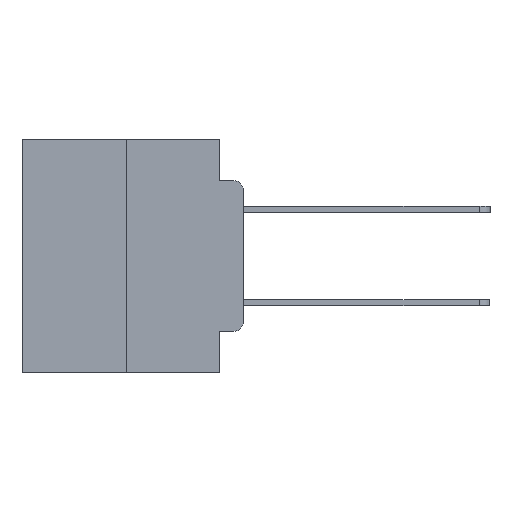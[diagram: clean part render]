
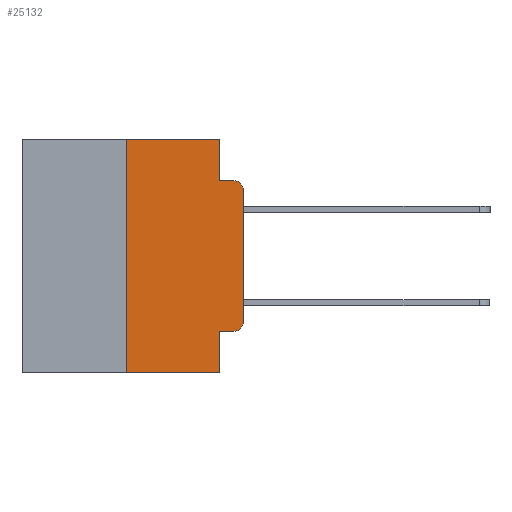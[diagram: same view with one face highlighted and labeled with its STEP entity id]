
A CAD part, left-side view. The second image highlights one B-rep face of the part: STEP entity #25132.
In plain terms, the highlighted planar face has unit normal (-1, 0, 0).
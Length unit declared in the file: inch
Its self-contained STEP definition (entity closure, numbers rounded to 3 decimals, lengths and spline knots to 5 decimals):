
#66 = CARTESIAN_POINT ( 'NONE',  ( 0., 0.051, -0.5 ) ) ;
#108 = CARTESIAN_POINT ( 'NONE',  ( 0., 0.02, -0.1085 ) ) ;
#1156 = ORIENTED_EDGE ( 'NONE', *, *, #16213, .T. ) ;
#1278 = FACE_OUTER_BOUND ( 'NONE', #3934, .T. ) ;
#1354 = VECTOR ( 'NONE', #22344, 39.37008 ) ;
#2232 = VECTOR ( 'NONE', #16869, 39.37008 ) ;
#2329 = DIRECTION ( 'NONE',  ( 0., 0., -1. ) ) ;
#2457 = EDGE_CURVE ( 'NONE', #13263, #21846, #18637, .T. ) ;
#3213 = CARTESIAN_POINT ( 'NONE',  ( 0., 0.02, -0.3915 ) ) ;
#3275 = CARTESIAN_POINT ( 'NONE',  ( 0., 0.051, -0.4115 ) ) ;
#3934 = EDGE_LOOP ( 'NONE', ( #9093, #15205, #4884, #15850, #16503, #17152, #1156, #7487, #18450, #19098 ) ) ;
#4312 = CIRCLE ( 'NONE', #15106, 0.02 ) ;
#4454 = CARTESIAN_POINT ( 'NONE',  ( 0., 0.25, -0.5 ) ) ;
#4498 = DIRECTION ( 'NONE',  ( 0., 0., 1. ) ) ;
#4884 = ORIENTED_EDGE ( 'NONE', *, *, #15669, .F. ) ;
#5142 = CARTESIAN_POINT ( 'NONE',  ( 0., 0., 0. ) ) ;
#5264 = CARTESIAN_POINT ( 'NONE',  ( 0., 0.473, -0.5 ) ) ;
#5349 = DIRECTION ( 'NONE',  ( 0., 0., -1. ) ) ;
#5828 = VERTEX_POINT ( 'NONE', #8620 ) ;
#6153 = DIRECTION ( 'NONE',  ( 0., -1., 0. ) ) ;
#6256 = CIRCLE ( 'NONE', #11082, 0.02 ) ;
#6885 = EDGE_CURVE ( 'NONE', #24458, #19609, #12962, .T. ) ;
#7334 = VECTOR ( 'NONE', #21661, 39.37008 ) ;
#7487 = ORIENTED_EDGE ( 'NONE', *, *, #10504, .F. ) ;
#7636 = CARTESIAN_POINT ( 'NONE',  ( 0., 0.051, -0.0885 ) ) ;
#7838 = LINE ( 'NONE', #25071, #2232 ) ;
#8212 = EDGE_CURVE ( 'NONE', #26313, #9872, #26751, .T. ) ;
#8465 = DIRECTION ( 'NONE',  ( 0., -1., 0. ) ) ;
#8620 = CARTESIAN_POINT ( 'NONE',  ( 0., 0.02, -0.0885 ) ) ;
#8842 = VERTEX_POINT ( 'NONE', #4454 ) ;
#8914 = VECTOR ( 'NONE', #21525, 39.37008 ) ;
#9093 = ORIENTED_EDGE ( 'NONE', *, *, #6885, .T. ) ;
#9577 = LINE ( 'NONE', #21605, #8914 ) ;
#9722 = DIRECTION ( 'NONE',  ( 0., 0., -1. ) ) ;
#9872 = VERTEX_POINT ( 'NONE', #20114 ) ;
#10504 = EDGE_CURVE ( 'NONE', #26313, #12236, #9577, .T. ) ;
#10576 = CARTESIAN_POINT ( 'NONE',  ( 0., 0.051, 0. ) ) ;
#10893 = CARTESIAN_POINT ( 'NONE',  ( 0., 0., -0.3915 ) ) ;
#11082 = AXIS2_PLACEMENT_3D ( 'NONE', #108, #14784, #2329 ) ;
#12236 = VERTEX_POINT ( 'NONE', #66 ) ;
#12962 = LINE ( 'NONE', #5142, #23252 ) ;
#13263 = VERTEX_POINT ( 'NONE', #14374 ) ;
#13465 = LINE ( 'NONE', #5264, #7334 ) ;
#14132 = VECTOR ( 'NONE', #6153, 39.37008 ) ;
#14374 = CARTESIAN_POINT ( 'NONE',  ( 0., 0.25, 0. ) ) ;
#14784 = DIRECTION ( 'NONE',  ( -1., 0., 0. ) ) ;
#15106 = AXIS2_PLACEMENT_3D ( 'NONE', #3213, #17707, #5349 ) ;
#15205 = ORIENTED_EDGE ( 'NONE', *, *, #19823, .T. ) ;
#15669 = EDGE_CURVE ( 'NONE', #20827, #5828, #19611, .T. ) ;
#15828 = CARTESIAN_POINT ( 'NONE',  ( 0., 0.473, 0. ) ) ;
#15850 = ORIENTED_EDGE ( 'NONE', *, *, #22575, .F. ) ;
#16065 = CARTESIAN_POINT ( 'NONE',  ( 0., 0., -0.1085 ) ) ;
#16116 = LINE ( 'NONE', #23200, #25789 ) ;
#16213 = EDGE_CURVE ( 'NONE', #8842, #12236, #13465, .T. ) ;
#16503 = ORIENTED_EDGE ( 'NONE', *, *, #2457, .F. ) ;
#16869 = DIRECTION ( 'NONE',  ( 0., 0., 1. ) ) ;
#17087 = DIRECTION ( 'NONE',  ( 0., 0., -1. ) ) ;
#17152 = ORIENTED_EDGE ( 'NONE', *, *, #18445, .F. ) ;
#17537 = AXIS2_PLACEMENT_3D ( 'NONE', #15828, #22033, #9722 ) ;
#17707 = DIRECTION ( 'NONE',  ( -1., 0., 0. ) ) ;
#18244 = CARTESIAN_POINT ( 'NONE',  ( 0., 0.473, 0. ) ) ;
#18445 = EDGE_CURVE ( 'NONE', #8842, #13263, #7838, .T. ) ;
#18450 = ORIENTED_EDGE ( 'NONE', *, *, #8212, .T. ) ;
#18637 = LINE ( 'NONE', #18244, #1354 ) ;
#19098 = ORIENTED_EDGE ( 'NONE', *, *, #25651, .T. ) ;
#19609 = VERTEX_POINT ( 'NONE', #16065 ) ;
#19611 = LINE ( 'NONE', #22539, #14132 ) ;
#19823 = EDGE_CURVE ( 'NONE', #19609, #5828, #6256, .T. ) ;
#19987 = PLANE ( 'NONE',  #17537 ) ;
#20114 = CARTESIAN_POINT ( 'NONE',  ( 0., 0.02, -0.4115 ) ) ;
#20827 = VERTEX_POINT ( 'NONE', #7636 ) ;
#20830 = CARTESIAN_POINT ( 'NONE',  ( 0., 0.051, -0.4115 ) ) ;
#21525 = DIRECTION ( 'NONE',  ( 0., 0., -1. ) ) ;
#21605 = CARTESIAN_POINT ( 'NONE',  ( 0., 0.051, 0. ) ) ;
#21661 = DIRECTION ( 'NONE',  ( 0., -1., 0. ) ) ;
#21846 = VERTEX_POINT ( 'NONE', #10576 ) ;
#22033 = DIRECTION ( 'NONE',  ( 1., 0., 0. ) ) ;
#22344 = DIRECTION ( 'NONE',  ( 0., -1., 0. ) ) ;
#22539 = CARTESIAN_POINT ( 'NONE',  ( 0., 0.051, -0.0885 ) ) ;
#22575 = EDGE_CURVE ( 'NONE', #21846, #20827, #16116, .T. ) ;
#23200 = CARTESIAN_POINT ( 'NONE',  ( 0., 0.051, 0. ) ) ;
#23252 = VECTOR ( 'NONE', #4498, 39.37008 ) ;
#24458 = VERTEX_POINT ( 'NONE', #10893 ) ;
#25071 = CARTESIAN_POINT ( 'NONE',  ( 0., 0.25, 0. ) ) ;
#25132 = ADVANCED_FACE ( 'NONE', ( #1278 ), #19987, .F. ) ;
#25651 = EDGE_CURVE ( 'NONE', #9872, #24458, #4312, .T. ) ;
#25789 = VECTOR ( 'NONE', #17087, 39.37008 ) ;
#26118 = VECTOR ( 'NONE', #8465, 39.37008 ) ;
#26313 = VERTEX_POINT ( 'NONE', #3275 ) ;
#26751 = LINE ( 'NONE', #20830, #26118 ) ;
